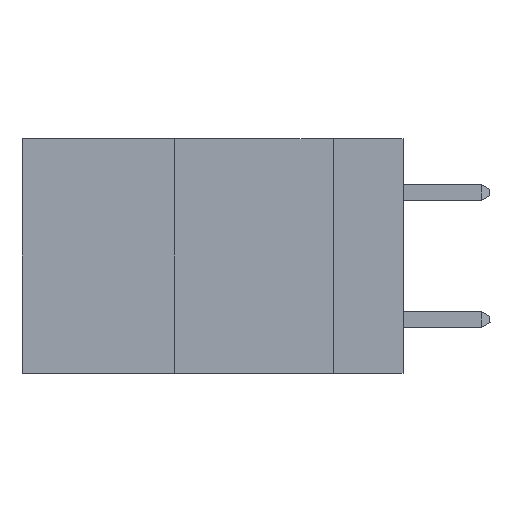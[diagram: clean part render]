
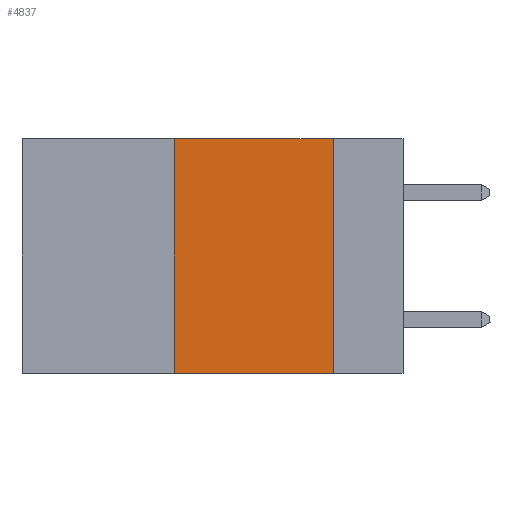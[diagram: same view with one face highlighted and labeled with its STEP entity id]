
A CAD part, left-side view. The second image highlights one B-rep face of the part: STEP entity #4837.
In plain terms, the highlighted planar face has unit normal (-1, 0, 0).
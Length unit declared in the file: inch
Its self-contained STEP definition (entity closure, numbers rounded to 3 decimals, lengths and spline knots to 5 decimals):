
#133 = VERTEX_POINT ( 'NONE', #11065 ) ;
#422 = CARTESIAN_POINT ( 'NONE',  ( 0., 0.36, 0. ) ) ;
#747 = VECTOR ( 'NONE', #8444, 39.37008 ) ;
#781 = ORIENTED_EDGE ( 'NONE', *, *, #11880, .F. ) ;
#890 = VERTEX_POINT ( 'NONE', #422 ) ;
#1008 = DIRECTION ( 'NONE',  ( 0., 0., -1. ) ) ;
#2015 = CARTESIAN_POINT ( 'NONE',  ( 0., 0.11, 0. ) ) ;
#2108 = EDGE_CURVE ( 'NONE', #890, #4439, #2823, .T. ) ;
#2543 = DIRECTION ( 'NONE',  ( 0., 0., 1. ) ) ;
#2615 = VECTOR ( 'NONE', #7740, 39.37008 ) ;
#2823 = LINE ( 'NONE', #6552, #747 ) ;
#4076 = VERTEX_POINT ( 'NONE', #10005 ) ;
#4439 = VERTEX_POINT ( 'NONE', #2015 ) ;
#4660 = VECTOR ( 'NONE', #2543, 39.37008 ) ;
#4837 = ADVANCED_FACE ( 'NONE', ( #10805 ), #11619, .F. ) ;
#5082 = CARTESIAN_POINT ( 'NONE',  ( 0., 0.6, -0.37 ) ) ;
#5156 = EDGE_CURVE ( 'NONE', #4439, #133, #6449, .T. ) ;
#5392 = DIRECTION ( 'NONE',  ( 1., 0., 0. ) ) ;
#5697 = CARTESIAN_POINT ( 'NONE',  ( 0., 0.11, 0. ) ) ;
#5925 = CARTESIAN_POINT ( 'NONE',  ( 0., 0.6, 0. ) ) ;
#6316 = VECTOR ( 'NONE', #1008, 39.37008 ) ;
#6449 = LINE ( 'NONE', #5697, #6316 ) ;
#6552 = CARTESIAN_POINT ( 'NONE',  ( 0., 0.6, 0. ) ) ;
#7205 = LINE ( 'NONE', #5082, #2615 ) ;
#7336 = AXIS2_PLACEMENT_3D ( 'NONE', #5925, #5392, #12236 ) ;
#7616 = ORIENTED_EDGE ( 'NONE', *, *, #9336, .T. ) ;
#7740 = DIRECTION ( 'NONE',  ( 0., -1., 0. ) ) ;
#7885 = LINE ( 'NONE', #9146, #4660 ) ;
#8444 = DIRECTION ( 'NONE',  ( 0., -1., 0. ) ) ;
#9146 = CARTESIAN_POINT ( 'NONE',  ( 0., 0.36, 0. ) ) ;
#9336 = EDGE_CURVE ( 'NONE', #4076, #133, #7205, .T. ) ;
#9580 = ORIENTED_EDGE ( 'NONE', *, *, #5156, .F. ) ;
#10005 = CARTESIAN_POINT ( 'NONE',  ( 0., 0.36, -0.37 ) ) ;
#10805 = FACE_OUTER_BOUND ( 'NONE', #10930, .T. ) ;
#10930 = EDGE_LOOP ( 'NONE', ( #9580, #11180, #781, #7616 ) ) ;
#11065 = CARTESIAN_POINT ( 'NONE',  ( 0., 0.11, -0.37 ) ) ;
#11180 = ORIENTED_EDGE ( 'NONE', *, *, #2108, .F. ) ;
#11619 = PLANE ( 'NONE',  #7336 ) ;
#11880 = EDGE_CURVE ( 'NONE', #4076, #890, #7885, .T. ) ;
#12236 = DIRECTION ( 'NONE',  ( 0., 0., -1. ) ) ;
